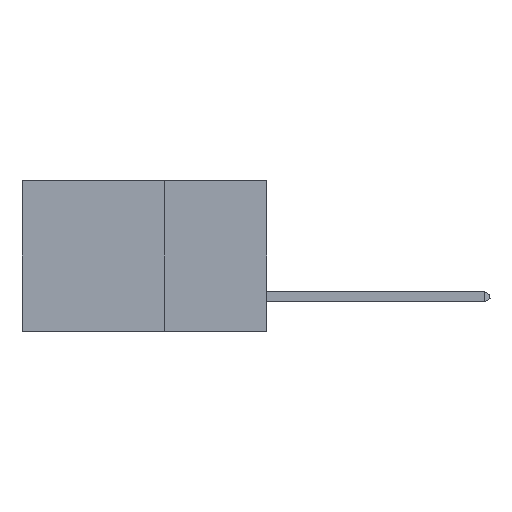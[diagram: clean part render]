
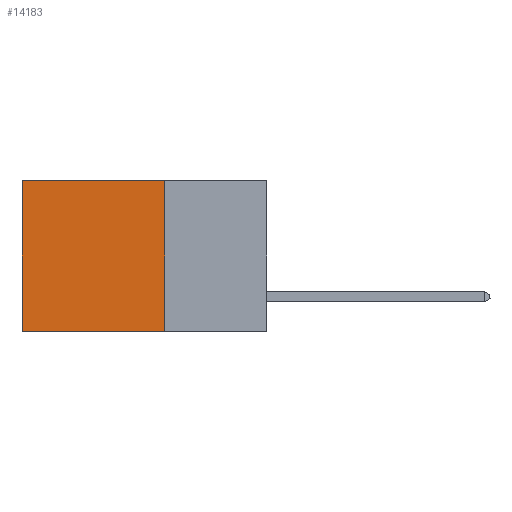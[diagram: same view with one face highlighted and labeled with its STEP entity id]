
A CAD part, left-side view. The second image highlights one B-rep face of the part: STEP entity #14183.
In plain terms, the highlighted planar face has unit normal (-1, 0, 0).
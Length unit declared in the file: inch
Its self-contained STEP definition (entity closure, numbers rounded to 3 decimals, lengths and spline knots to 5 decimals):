
#146 = EDGE_CURVE ( 'NONE', #682, #21008, #17368, .T. ) ;
#549 = CARTESIAN_POINT ( 'NONE',  ( 0.2875, 0.6, -0.37 ) ) ;
#669 = FACE_OUTER_BOUND ( 'NONE', #14431, .T. ) ;
#682 = VERTEX_POINT ( 'NONE', #16032 ) ;
#990 = PLANE ( 'NONE',  #8658 ) ;
#1040 = LINE ( 'NONE', #2128, #17840 ) ;
#1277 = EDGE_CURVE ( 'NONE', #19894, #21008, #1040, .T. ) ;
#1540 = ORIENTED_EDGE ( 'NONE', *, *, #146, .F. ) ;
#1602 = VECTOR ( 'NONE', #8001, 39.37008 ) ;
#2128 = CARTESIAN_POINT ( 'NONE',  ( 0.2875, 0.6, 0. ) ) ;
#4345 = VECTOR ( 'NONE', #7916, 39.37008 ) ;
#4479 = CARTESIAN_POINT ( 'NONE',  ( 0.2875, 0.25, 0. ) ) ;
#4488 = ORIENTED_EDGE ( 'NONE', *, *, #1277, .T. ) ;
#4941 = CARTESIAN_POINT ( 'NONE',  ( 0.2875, 0.6, 0. ) ) ;
#6835 = CARTESIAN_POINT ( 'NONE',  ( 0.2875, 0.25, 0. ) ) ;
#7916 = DIRECTION ( 'NONE',  ( 0., 0., -1. ) ) ;
#8001 = DIRECTION ( 'NONE',  ( 0., 1., 0. ) ) ;
#8658 = AXIS2_PLACEMENT_3D ( 'NONE', #4479, #19064, #9191 ) ;
#8721 = LINE ( 'NONE', #15838, #4345 ) ;
#9191 = DIRECTION ( 'NONE',  ( 0., 0., -1. ) ) ;
#10777 = LINE ( 'NONE', #6835, #11010 ) ;
#11010 = VECTOR ( 'NONE', #14980, 39.37008 ) ;
#12102 = EDGE_CURVE ( 'NONE', #14289, #682, #8721, .T. ) ;
#14183 = ADVANCED_FACE ( 'NONE', ( #669 ), #990, .F. ) ;
#14289 = VERTEX_POINT ( 'NONE', #14684 ) ;
#14431 = EDGE_LOOP ( 'NONE', ( #4488, #1540, #20802, #20630 ) ) ;
#14684 = CARTESIAN_POINT ( 'NONE',  ( 0.2875, 0.25, 0. ) ) ;
#14980 = DIRECTION ( 'NONE',  ( 0., 1., 0. ) ) ;
#15072 = DIRECTION ( 'NONE',  ( 0., 0., -1. ) ) ;
#15838 = CARTESIAN_POINT ( 'NONE',  ( 0.2875, 0.25, 0. ) ) ;
#16032 = CARTESIAN_POINT ( 'NONE',  ( 0.2875, 0.25, -0.37 ) ) ;
#17368 = LINE ( 'NONE', #17688, #1602 ) ;
#17688 = CARTESIAN_POINT ( 'NONE',  ( 0.2875, 0.25, -0.37 ) ) ;
#17840 = VECTOR ( 'NONE', #15072, 39.37008 ) ;
#19064 = DIRECTION ( 'NONE',  ( 1., 0., 0. ) ) ;
#19463 = EDGE_CURVE ( 'NONE', #14289, #19894, #10777, .T. ) ;
#19894 = VERTEX_POINT ( 'NONE', #4941 ) ;
#20630 = ORIENTED_EDGE ( 'NONE', *, *, #19463, .T. ) ;
#20802 = ORIENTED_EDGE ( 'NONE', *, *, #12102, .F. ) ;
#21008 = VERTEX_POINT ( 'NONE', #549 ) ;
